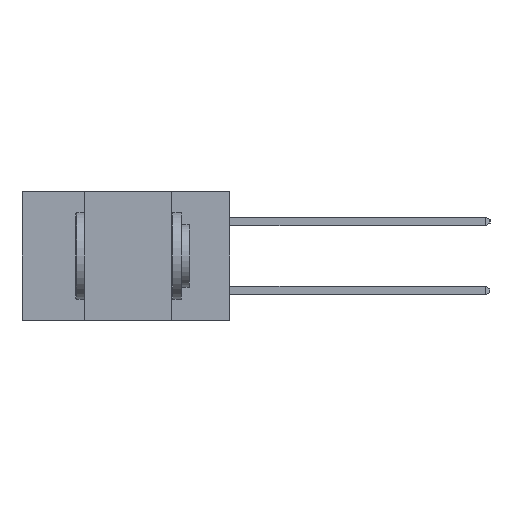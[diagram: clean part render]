
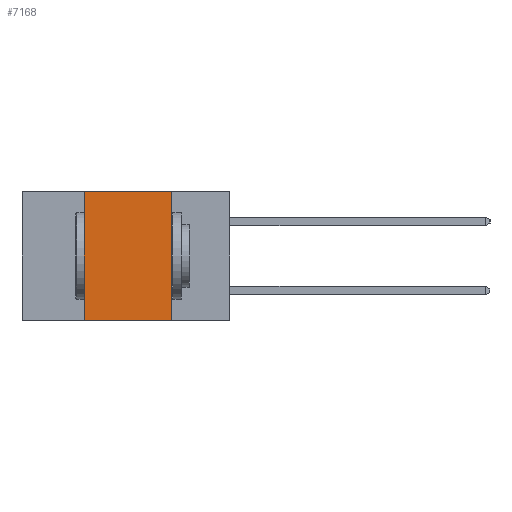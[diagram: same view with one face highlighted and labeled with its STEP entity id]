
A CAD part, left-side view. The second image highlights one B-rep face of the part: STEP entity #7168.
In plain terms, the highlighted planar face has unit normal (-1, 0, 0).
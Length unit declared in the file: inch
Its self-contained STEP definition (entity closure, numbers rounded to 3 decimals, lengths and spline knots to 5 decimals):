
#249 = CARTESIAN_POINT ( 'NONE',  ( 0., 0.17, -0.37 ) ) ;
#1117 = ORIENTED_EDGE ( 'NONE', *, *, #9128, .T. ) ;
#1548 = DIRECTION ( 'NONE',  ( 0., 0., 1. ) ) ;
#2138 = CARTESIAN_POINT ( 'NONE',  ( 0., 0.6, 0. ) ) ;
#3086 = CARTESIAN_POINT ( 'NONE',  ( 0., 0.6, -0.37 ) ) ;
#3680 = DIRECTION ( 'NONE',  ( 1., 0., 0. ) ) ;
#4172 = LINE ( 'NONE', #249, #26213 ) ;
#4345 = DIRECTION ( 'NONE',  ( 0., -1., 0. ) ) ;
#5520 = ORIENTED_EDGE ( 'NONE', *, *, #27221, .F. ) ;
#5762 = LINE ( 'NONE', #3086, #22171 ) ;
#7168 = ADVANCED_FACE ( 'NONE', ( #25532 ), #14505, .F. ) ;
#7695 = VERTEX_POINT ( 'NONE', #20388 ) ;
#9128 = EDGE_CURVE ( 'NONE', #19823, #7695, #5762, .T. ) ;
#9284 = CARTESIAN_POINT ( 'NONE',  ( 0., 0.17, 0. ) ) ;
#9818 = VECTOR ( 'NONE', #4345, 39.37008 ) ;
#10237 = CARTESIAN_POINT ( 'NONE',  ( 0., 0.42, -0.37 ) ) ;
#11058 = CARTESIAN_POINT ( 'NONE',  ( 0., 0.42, -0.37 ) ) ;
#11634 = VECTOR ( 'NONE', #1548, 39.37008 ) ;
#12368 = CARTESIAN_POINT ( 'NONE',  ( 0., 0.6, 0. ) ) ;
#14505 = PLANE ( 'NONE',  #20983 ) ;
#16368 = VERTEX_POINT ( 'NONE', #27452 ) ;
#16619 = LINE ( 'NONE', #10237, #11634 ) ;
#18188 = DIRECTION ( 'NONE',  ( 0., -1., 0. ) ) ;
#18754 = DIRECTION ( 'NONE',  ( 0., 0., -1. ) ) ;
#19688 = DIRECTION ( 'NONE',  ( 0., 0., -1. ) ) ;
#19823 = VERTEX_POINT ( 'NONE', #11058 ) ;
#20388 = CARTESIAN_POINT ( 'NONE',  ( 0., 0.17, -0.37 ) ) ;
#20983 = AXIS2_PLACEMENT_3D ( 'NONE', #12368, #3680, #18754 ) ;
#21188 = VERTEX_POINT ( 'NONE', #9284 ) ;
#22171 = VECTOR ( 'NONE', #18188, 39.37008 ) ;
#22873 = EDGE_CURVE ( 'NONE', #19823, #16368, #16619, .T. ) ;
#24492 = EDGE_CURVE ( 'NONE', #16368, #21188, #26705, .T. ) ;
#25532 = FACE_OUTER_BOUND ( 'NONE', #27593, .T. ) ;
#25710 = ORIENTED_EDGE ( 'NONE', *, *, #22873, .F. ) ;
#26213 = VECTOR ( 'NONE', #19688, 39.37008 ) ;
#26705 = LINE ( 'NONE', #2138, #9818 ) ;
#27221 = EDGE_CURVE ( 'NONE', #21188, #7695, #4172, .T. ) ;
#27452 = CARTESIAN_POINT ( 'NONE',  ( 0., 0.42, 0. ) ) ;
#27593 = EDGE_LOOP ( 'NONE', ( #5520, #27629, #25710, #1117 ) ) ;
#27629 = ORIENTED_EDGE ( 'NONE', *, *, #24492, .F. ) ;
